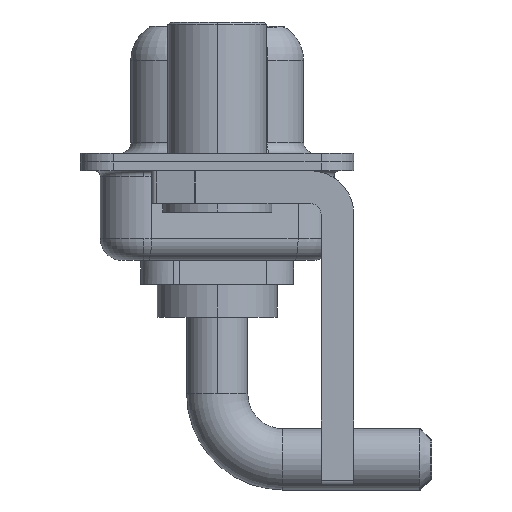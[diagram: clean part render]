
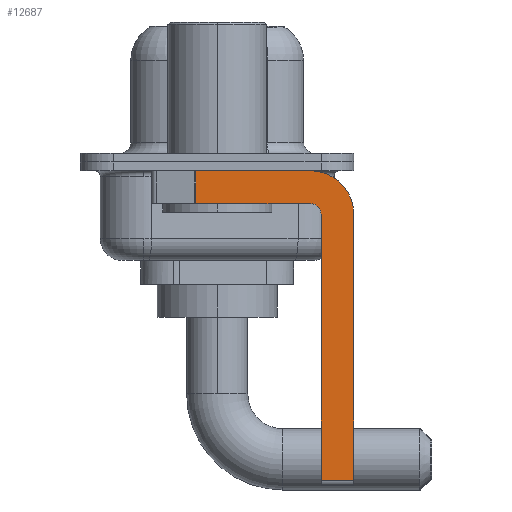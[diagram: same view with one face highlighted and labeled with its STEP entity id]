
A CAD part, left-side view. The second image highlights one B-rep face of the part: STEP entity #12687.
In plain terms, the highlighted planar face has unit normal (-1, 0, 0).
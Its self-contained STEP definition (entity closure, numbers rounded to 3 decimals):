
#105 = VERTEX_POINT ( 'NONE', #780 ) ;
#661 = ORIENTED_EDGE ( 'NONE', *, *, #6364, .F. ) ;
#780 = CARTESIAN_POINT ( 'NONE',  ( -2.9, -4.25, -0.4 ) ) ;
#795 = ORIENTED_EDGE ( 'NONE', *, *, #1298, .T. ) ;
#1097 = CARTESIAN_POINT ( 'NONE',  ( -2.9, -4.75, -14.8 ) ) ;
#1192 = DIRECTION ( 'NONE',  ( 0., 0., 1. ) ) ;
#1298 = EDGE_CURVE ( 'NONE', #9998, #13338, #13565, .T. ) ;
#1368 = VERTEX_POINT ( 'NONE', #4816 ) ;
#1458 = CIRCLE ( 'NONE', #11462, 0.5 ) ;
#1560 = VECTOR ( 'NONE', #15121, 1000. ) ;
#1613 = VERTEX_POINT ( 'NONE', #14449 ) ;
#2015 = ORIENTED_EDGE ( 'NONE', *, *, #11255, .F. ) ;
#2198 = PLANE ( 'NONE',  #8385 ) ;
#2446 = DIRECTION ( 'NONE',  ( -1., 0., 0. ) ) ;
#2522 = DIRECTION ( 'NONE',  ( 0., 0., -1. ) ) ;
#2681 = CARTESIAN_POINT ( 'NONE',  ( -2.9, -4.75, -14.55 ) ) ;
#3555 = VECTOR ( 'NONE', #6186, 1000. ) ;
#4393 = DIRECTION ( 'NONE',  ( 0., -1., 0. ) ) ;
#4661 = FACE_OUTER_BOUND ( 'NONE', #4953, .T. ) ;
#4774 = VECTOR ( 'NONE', #14878, 1000. ) ;
#4816 = CARTESIAN_POINT ( 'NONE',  ( -2.9, -4.75, -2.4 ) ) ;
#4953 = EDGE_LOOP ( 'NONE', ( #8363, #14349, #6493, #14565, #661, #795, #2015, #8327 ) ) ;
#5048 = LINE ( 'NONE', #8902, #1560 ) ;
#5173 = CARTESIAN_POINT ( 'NONE',  ( -2.9, -4.25, -2.4 ) ) ;
#5250 = DIRECTION ( 'NONE',  ( 0., 0., -1. ) ) ;
#5317 = CARTESIAN_POINT ( 'NONE',  ( -2.9, 0.978, -1.9 ) ) ;
#5934 = VECTOR ( 'NONE', #11491, 1000. ) ;
#5998 = EDGE_CURVE ( 'NONE', #1613, #14441, #9928, .T. ) ;
#6057 = EDGE_CURVE ( 'NONE', #1368, #1613, #1458, .T. ) ;
#6186 = DIRECTION ( 'NONE',  ( 0., 0., 1. ) ) ;
#6195 = VERTEX_POINT ( 'NONE', #9174 ) ;
#6288 = CARTESIAN_POINT ( 'NONE',  ( -2.9, -6.25, -2.4 ) ) ;
#6364 = EDGE_CURVE ( 'NONE', #9998, #1368, #11309, .T. ) ;
#6493 = ORIENTED_EDGE ( 'NONE', *, *, #5998, .F. ) ;
#7021 = VECTOR ( 'NONE', #4393, 1000. ) ;
#8252 = CARTESIAN_POINT ( 'NONE',  ( -2.9, -4.25, -14.55 ) ) ;
#8327 = ORIENTED_EDGE ( 'NONE', *, *, #13808, .F. ) ;
#8363 = ORIENTED_EDGE ( 'NONE', *, *, #11672, .F. ) ;
#8385 = AXIS2_PLACEMENT_3D ( 'NONE', #14737, #13247, #11922 ) ;
#8693 = CARTESIAN_POINT ( 'NONE',  ( -2.9, -4.25, -2.4 ) ) ;
#8774 = CARTESIAN_POINT ( 'NONE',  ( -2.9, -6.25, -2.4 ) ) ;
#8902 = CARTESIAN_POINT ( 'NONE',  ( -2.9, 0.978, -1.9 ) ) ;
#8923 = AXIS2_PLACEMENT_3D ( 'NONE', #5173, #9954, #5250 ) ;
#8941 = EDGE_CURVE ( 'NONE', #6195, #14441, #5048, .T. ) ;
#9174 = CARTESIAN_POINT ( 'NONE',  ( -2.9, 0.978, -0.4 ) ) ;
#9763 = VERTEX_POINT ( 'NONE', #8774 ) ;
#9928 = LINE ( 'NONE', #12664, #5934 ) ;
#9954 = DIRECTION ( 'NONE',  ( 1., 0., 0. ) ) ;
#9998 = VERTEX_POINT ( 'NONE', #2681 ) ;
#11255 = EDGE_CURVE ( 'NONE', #9763, #13338, #12666, .T. ) ;
#11309 = LINE ( 'NONE', #1097, #3555 ) ;
#11462 = AXIS2_PLACEMENT_3D ( 'NONE', #8693, #2446, #1192 ) ;
#11491 = DIRECTION ( 'NONE',  ( 0., 1., 0. ) ) ;
#11565 = CIRCLE ( 'NONE', #8923, 2. ) ;
#11672 = EDGE_CURVE ( 'NONE', #6195, #105, #15873, .T. ) ;
#11922 = DIRECTION ( 'NONE',  ( 0., 0., -1. ) ) ;
#12664 = CARTESIAN_POINT ( 'NONE',  ( -2.9, -4.25, -1.9 ) ) ;
#12666 = LINE ( 'NONE', #6288, #15739 ) ;
#12687 = ADVANCED_FACE ( 'NONE', ( #4661 ), #2198, .F. ) ;
#13247 = DIRECTION ( 'NONE',  ( 1., 0., 0. ) ) ;
#13338 = VERTEX_POINT ( 'NONE', #14114 ) ;
#13565 = LINE ( 'NONE', #8252, #4774 ) ;
#13808 = EDGE_CURVE ( 'NONE', #105, #9763, #11565, .T. ) ;
#14114 = CARTESIAN_POINT ( 'NONE',  ( -2.9, -6.25, -14.55 ) ) ;
#14349 = ORIENTED_EDGE ( 'NONE', *, *, #8941, .T. ) ;
#14441 = VERTEX_POINT ( 'NONE', #5317 ) ;
#14449 = CARTESIAN_POINT ( 'NONE',  ( -2.9, -4.25, -1.9 ) ) ;
#14565 = ORIENTED_EDGE ( 'NONE', *, *, #6057, .F. ) ;
#14737 = CARTESIAN_POINT ( 'NONE',  ( -2.9, -4.25, -2.4 ) ) ;
#14878 = DIRECTION ( 'NONE',  ( 0., -1., 0. ) ) ;
#15121 = DIRECTION ( 'NONE',  ( 0., 0., -1. ) ) ;
#15739 = VECTOR ( 'NONE', #2522, 1000. ) ;
#15873 = LINE ( 'NONE', #15952, #7021 ) ;
#15952 = CARTESIAN_POINT ( 'NONE',  ( -2.9, 3., -0.4 ) ) ;
